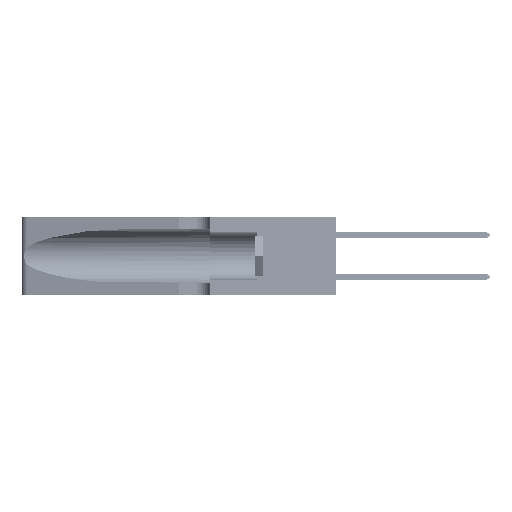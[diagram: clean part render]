
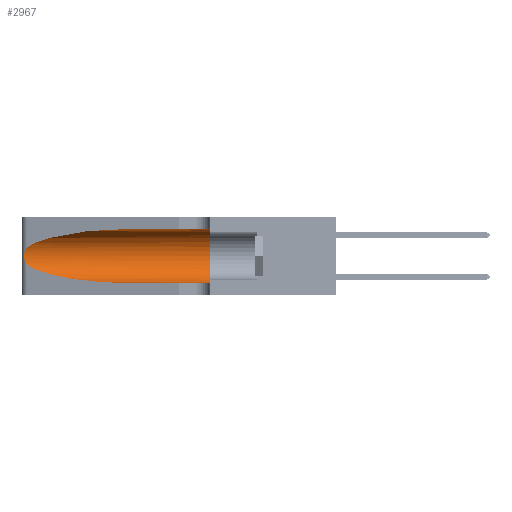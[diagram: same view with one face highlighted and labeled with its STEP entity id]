
A CAD part, left-side view. The second image highlights one B-rep face of the part: STEP entity #2967.
In plain terms, the highlighted cylindrical face has radius 3.308 mm (diameter 6.617 mm), a partial arc.
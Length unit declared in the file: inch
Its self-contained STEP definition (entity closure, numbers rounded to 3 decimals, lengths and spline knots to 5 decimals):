
#92 = EDGE_CURVE ( 'NONE', #45085, #31153, #14665, .T. ) ;
#285 = ORIENTED_EDGE ( 'NONE', *, *, #30913, .T. ) ;
#2967 = ADVANCED_FACE ( 'NONE', ( #6229 ), #14427, .F. ) ;
#3061 = CARTESIAN_POINT ( 'NONE',  ( 0.25789, 1.23486, 0.15765 ) ) ;
#3485 = CARTESIAN_POINT ( 'NONE',  ( 0.2373, 1.15595, 0.28018 ) ) ;
#3497 = VERTEX_POINT ( 'NONE', #4531 ) ;
#4090 = ORIENTED_EDGE ( 'NONE', *, *, #16372, .F. ) ;
#4531 = CARTESIAN_POINT ( 'NONE',  ( 0.1305, 0.72297, 0.05475 ) ) ;
#5432 = ORIENTED_EDGE ( 'NONE', *, *, #25696, .T. ) ;
#6179 = VERTEX_POINT ( 'NONE', #35464 ) ;
#6229 = FACE_OUTER_BOUND ( 'NONE', #25475, .T. ) ;
#6950 = CARTESIAN_POINT ( 'NONE',  ( 0.25487, 1.22718, 0.22369 ) ) ;
#7113 = CARTESIAN_POINT ( 'NONE',  ( 0.25555, 1.22993, 0.14849 ) ) ;
#7645 = VECTOR ( 'NONE', #8528, 39.37008 ) ;
#8342 = LINE ( 'NONE', #41025, #17847 ) ;
#8528 = DIRECTION ( 'NONE',  ( 0., -1., 0. ) ) ;
#9327 = ORIENTED_EDGE ( 'NONE', *, *, #92, .F. ) ;
#9843 = CARTESIAN_POINT ( 'NONE',  ( 0.25487, 1.22718, 0.14631 ) ) ;
#13019 = VERTEX_POINT ( 'NONE', #28388 ) ;
#14427 = CYLINDRICAL_SURFACE ( 'NONE', #47332, 0.13025 ) ;
#14665 = CIRCLE ( 'NONE', #44592, 0.13025 ) ;
#15066 = CARTESIAN_POINT ( 'NONE',  ( 0.25787, 1.23484, 0.2124 ) ) ;
#15699 =( BOUNDED_CURVE ( )  B_SPLINE_CURVE ( 3, ( #19567, #23639, #3485, #31674 ),
 .UNSPECIFIED., .F., .T. ) 
 B_SPLINE_CURVE_WITH_KNOTS ( ( 4, 4 ),
 ( 1.5708, 2.84003 ),
 .UNSPECIFIED. ) 
 CURVE ( )  GEOMETRIC_REPRESENTATION_ITEM ( )  RATIONAL_B_SPLINE_CURVE ( ( 1., 0.87, 0.87, 1. ) ) 
 REPRESENTATION_ITEM ( '' )  );
#16372 = EDGE_CURVE ( 'NONE', #19396, #45085, #8342, .T. ) ;
#17056 = EDGE_CURVE ( 'NONE', #3497, #31153, #51465, .T. ) ;
#17847 = VECTOR ( 'NONE', #45024, 39.37008 ) ;
#19146 = CARTESIAN_POINT ( 'NONE',  ( 0.26018, 1.23835, 0.19895 ) ) ;
#19396 = VERTEX_POINT ( 'NONE', #43192 ) ;
#19567 = CARTESIAN_POINT ( 'NONE',  ( 0.1305, 0.72297, 0.31525 ) ) ;
#20851 = DIRECTION ( 'NONE',  ( 0., 0., -1. ) ) ;
#22070 = CARTESIAN_POINT ( 'NONE',  ( 0.18966, 0.96281, 0.05475 ) ) ;
#22345 = CARTESIAN_POINT ( 'NONE',  ( 0.1305, 0.35, 0.185 ) ) ;
#23207 = CARTESIAN_POINT ( 'NONE',  ( 0.26075, 1.23896, 0.178 ) ) ;
#23639 = CARTESIAN_POINT ( 'NONE',  ( 0.18966, 0.96281, 0.31525 ) ) ;
#25475 = EDGE_LOOP ( 'NONE', ( #45709, #5432, #285, #41270, #9327, #4090 ) ) ;
#25696 = EDGE_CURVE ( 'NONE', #6179, #13019, #38194, .T. ) ;
#26379 = DIRECTION ( 'NONE',  ( 0., 0., 1. ) ) ;
#27240 = CARTESIAN_POINT ( 'NONE',  ( 0.25856, 1.23593, 0.16098 ) ) ;
#28388 = CARTESIAN_POINT ( 'NONE',  ( 0.25487, 1.22718, 0.14631 ) ) ;
#28928 =( BOUNDED_CURVE ( )  B_SPLINE_CURVE ( 3, ( #9843, #33971, #22070, #49876 ),
 .UNSPECIFIED., .F., .F. ) 
 B_SPLINE_CURVE_WITH_KNOTS ( ( 4, 4 ),
 ( 3.44316, 4.71239 ),
 .UNSPECIFIED. ) 
 CURVE ( )  GEOMETRIC_REPRESENTATION_ITEM ( )  RATIONAL_B_SPLINE_CURVE ( ( 1., 0.87, 0.87, 1. ) ) 
 REPRESENTATION_ITEM ( '' )  );
#29989 = CARTESIAN_POINT ( 'NONE',  ( 0.1305, 0.35, 0.31525 ) ) ;
#30913 = EDGE_CURVE ( 'NONE', #13019, #3497, #28928, .T. ) ;
#31081 = CARTESIAN_POINT ( 'NONE',  ( 0.25555, 1.22994, 0.2215 ) ) ;
#31153 = VERTEX_POINT ( 'NONE', #47436 ) ;
#31246 = CARTESIAN_POINT ( 'NONE',  ( 0.25639, 1.23186, 0.15144 ) ) ;
#31674 = CARTESIAN_POINT ( 'NONE',  ( 0.25487, 1.22718, 0.22369 ) ) ;
#33971 = CARTESIAN_POINT ( 'NONE',  ( 0.2373, 1.15595, 0.08982 ) ) ;
#35256 = CARTESIAN_POINT ( 'NONE',  ( 0.25487, 1.22718, 0.14631 ) ) ;
#35464 = CARTESIAN_POINT ( 'NONE',  ( 0.25487, 1.22718, 0.22369 ) ) ;
#36636 = CARTESIAN_POINT ( 'NONE',  ( 0.1305, 1.61858, 0.05475 ) ) ;
#36735 = CARTESIAN_POINT ( 'NONE',  ( 0.1305, 1.61858, 0.185 ) ) ;
#38194 = B_SPLINE_CURVE_WITH_KNOTS ( 'NONE', 3,
 ( #6950, #31081, #39074, #15066, #43053, #19146, #47051, #23207, #51019, #27240, #3061, #31246, #7113, #35256 ),
 .UNSPECIFIED., .F., .F.,
 ( 4, 2, 2, 2, 2, 2, 4 ),
 ( 0., 0.00027, 0.00053, 0.00107, 0.0016, 0.00187, 0.00214 ),
 .UNSPECIFIED. ) ;
#39074 = CARTESIAN_POINT ( 'NONE',  ( 0.25639, 1.23184, 0.21858 ) ) ;
#41025 = CARTESIAN_POINT ( 'NONE',  ( 0.1305, 1.61858, 0.31525 ) ) ;
#41270 = ORIENTED_EDGE ( 'NONE', *, *, #17056, .T. ) ;
#43053 = CARTESIAN_POINT ( 'NONE',  ( 0.25854, 1.2359, 0.20912 ) ) ;
#43192 = CARTESIAN_POINT ( 'NONE',  ( 0.1305, 0.72297, 0.31525 ) ) ;
#44592 = AXIS2_PLACEMENT_3D ( 'NONE', #22345, #50169, #26379 ) ;
#44705 = DIRECTION ( 'NONE',  ( 0., -1., 0. ) ) ;
#45024 = DIRECTION ( 'NONE',  ( 0., -1., 0. ) ) ;
#45085 = VERTEX_POINT ( 'NONE', #29989 ) ;
#45709 = ORIENTED_EDGE ( 'NONE', *, *, #49704, .T. ) ;
#47051 = CARTESIAN_POINT ( 'NONE',  ( 0.26075, 1.23896, 0.19203 ) ) ;
#47332 = AXIS2_PLACEMENT_3D ( 'NONE', #36735, #44705, #20851 ) ;
#47436 = CARTESIAN_POINT ( 'NONE',  ( 0.1305, 0.35, 0.05475 ) ) ;
#49704 = EDGE_CURVE ( 'NONE', #19396, #6179, #15699, .T. ) ;
#49876 = CARTESIAN_POINT ( 'NONE',  ( 0.1305, 0.72297, 0.05475 ) ) ;
#50169 = DIRECTION ( 'NONE',  ( 0., 1., 0. ) ) ;
#51019 = CARTESIAN_POINT ( 'NONE',  ( 0.26017, 1.23833, 0.17102 ) ) ;
#51465 = LINE ( 'NONE', #36636, #7645 ) ;
